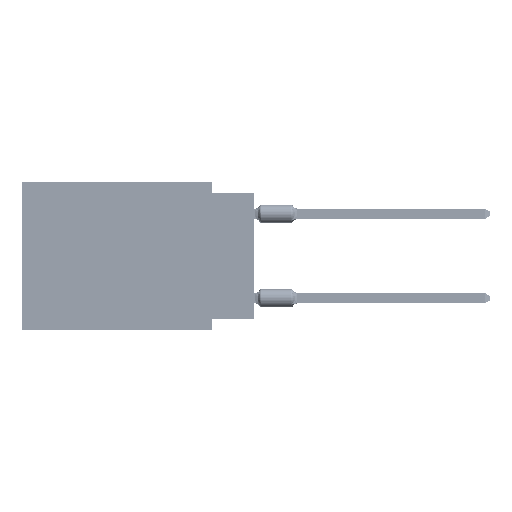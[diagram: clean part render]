
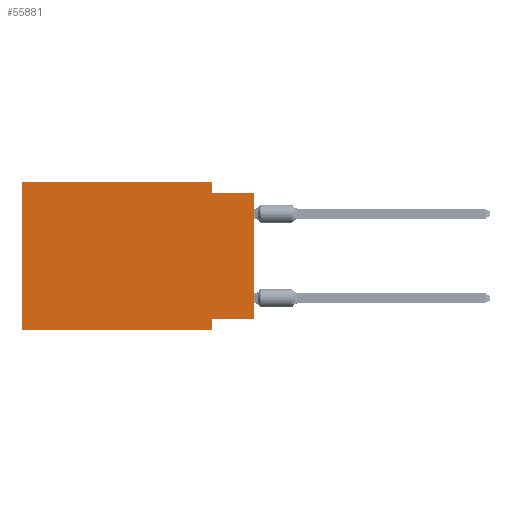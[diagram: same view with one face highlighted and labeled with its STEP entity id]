
A CAD part, left-side view. The second image highlights one B-rep face of the part: STEP entity #55881.
In plain terms, the highlighted planar face has unit normal (-1, 0, 0).
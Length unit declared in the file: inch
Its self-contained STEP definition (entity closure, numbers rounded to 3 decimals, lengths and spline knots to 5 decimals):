
#1097 = LINE ( 'NONE', #75760, #68045 ) ;
#5386 = LINE ( 'NONE', #37117, #77578 ) ;
#5745 = CARTESIAN_POINT ( 'NONE',  ( 0., 0., -0.325 ) ) ;
#5832 = DIRECTION ( 'NONE',  ( 0., 0., -1. ) ) ;
#6381 = LINE ( 'NONE', #80609, #19720 ) ;
#6536 = LINE ( 'NONE', #32493, #61028 ) ;
#7744 = ORIENTED_EDGE ( 'NONE', *, *, #44797, .F. ) ;
#8348 = LINE ( 'NONE', #50827, #13040 ) ;
#11417 = VECTOR ( 'NONE', #65275, 39.37008 ) ;
#11890 = VECTOR ( 'NONE', #18462, 39.37008 ) ;
#12541 = VERTEX_POINT ( 'NONE', #80105 ) ;
#12855 = VERTEX_POINT ( 'NONE', #28084 ) ;
#13040 = VECTOR ( 'NONE', #76404, 39.37008 ) ;
#14979 = CARTESIAN_POINT ( 'NONE',  ( 0., 0.55, 0. ) ) ;
#15381 = ORIENTED_EDGE ( 'NONE', *, *, #74983, .F. ) ;
#15388 = AXIS2_PLACEMENT_3D ( 'NONE', #56130, #63106, #5832 ) ;
#16599 = VERTEX_POINT ( 'NONE', #37852 ) ;
#17278 = ORIENTED_EDGE ( 'NONE', *, *, #69073, .T. ) ;
#18462 = DIRECTION ( 'NONE',  ( 0., 0., -1. ) ) ;
#18869 = LINE ( 'NONE', #69565, #11890 ) ;
#19720 = VECTOR ( 'NONE', #30726, 39.37008 ) ;
#26302 = CARTESIAN_POINT ( 'NONE',  ( 0., 0.1, 0. ) ) ;
#26573 = EDGE_CURVE ( 'NONE', #48673, #60899, #77673, .T. ) ;
#28084 = CARTESIAN_POINT ( 'NONE',  ( 0., 0.1, -0.35 ) ) ;
#29570 = CARTESIAN_POINT ( 'NONE',  ( 0., 0.1, -0.025 ) ) ;
#30726 = DIRECTION ( 'NONE',  ( 0., 1., 0. ) ) ;
#32493 = CARTESIAN_POINT ( 'NONE',  ( 0., 0., 0. ) ) ;
#32502 = EDGE_CURVE ( 'NONE', #16599, #12855, #18869, .T. ) ;
#36100 = ORIENTED_EDGE ( 'NONE', *, *, #45724, .F. ) ;
#37117 = CARTESIAN_POINT ( 'NONE',  ( 0., 0.55, 0. ) ) ;
#37852 = CARTESIAN_POINT ( 'NONE',  ( 0., 0.1, -0.325 ) ) ;
#39612 = ORIENTED_EDGE ( 'NONE', *, *, #26573, .F. ) ;
#44237 = VECTOR ( 'NONE', #76610, 39.37008 ) ;
#44797 = EDGE_CURVE ( 'NONE', #57506, #16599, #6381, .T. ) ;
#45233 = LINE ( 'NONE', #26302, #44237 ) ;
#45724 = EDGE_CURVE ( 'NONE', #60899, #12541, #5386, .T. ) ;
#47820 = ORIENTED_EDGE ( 'NONE', *, *, #32502, .F. ) ;
#48673 = VERTEX_POINT ( 'NONE', #66252 ) ;
#48918 = CARTESIAN_POINT ( 'NONE',  ( 0., 0.55, 0. ) ) ;
#50827 = CARTESIAN_POINT ( 'NONE',  ( 0., 0.55, -0.35 ) ) ;
#51404 = DIRECTION ( 'NONE',  ( 0., -1., 0. ) ) ;
#53698 = VERTEX_POINT ( 'NONE', #29570 ) ;
#54757 = EDGE_CURVE ( 'NONE', #12541, #53698, #45233, .T. ) ;
#55881 = ADVANCED_FACE ( 'NONE', ( #75900 ), #63513, .F. ) ;
#56130 = CARTESIAN_POINT ( 'NONE',  ( 0., 0.55, 0. ) ) ;
#56326 = EDGE_LOOP ( 'NONE', ( #17278, #15381, #77505, #36100, #39612, #61687, #47820, #7744 ) ) ;
#57506 = VERTEX_POINT ( 'NONE', #5745 ) ;
#58473 = EDGE_CURVE ( 'NONE', #48673, #12855, #8348, .T. ) ;
#60899 = VERTEX_POINT ( 'NONE', #48918 ) ;
#61028 = VECTOR ( 'NONE', #77417, 39.37008 ) ;
#61687 = ORIENTED_EDGE ( 'NONE', *, *, #58473, .T. ) ;
#63106 = DIRECTION ( 'NONE',  ( 1., 0., 0. ) ) ;
#63513 = PLANE ( 'NONE',  #15388 ) ;
#65275 = DIRECTION ( 'NONE',  ( 0., 0., 1. ) ) ;
#65964 = VERTEX_POINT ( 'NONE', #77599 ) ;
#66252 = CARTESIAN_POINT ( 'NONE',  ( 0., 0.55, -0.35 ) ) ;
#68045 = VECTOR ( 'NONE', #51404, 39.37008 ) ;
#69073 = EDGE_CURVE ( 'NONE', #57506, #65964, #6536, .T. ) ;
#69565 = CARTESIAN_POINT ( 'NONE',  ( 0., 0.1, -0.35 ) ) ;
#74983 = EDGE_CURVE ( 'NONE', #53698, #65964, #1097, .T. ) ;
#75760 = CARTESIAN_POINT ( 'NONE',  ( 0., 0., -0.025 ) ) ;
#75900 = FACE_OUTER_BOUND ( 'NONE', #56326, .T. ) ;
#76404 = DIRECTION ( 'NONE',  ( 0., -1., 0. ) ) ;
#76610 = DIRECTION ( 'NONE',  ( 0., 0., -1. ) ) ;
#77417 = DIRECTION ( 'NONE',  ( 0., 0., 1. ) ) ;
#77505 = ORIENTED_EDGE ( 'NONE', *, *, #54757, .F. ) ;
#77578 = VECTOR ( 'NONE', #81240, 39.37008 ) ;
#77599 = CARTESIAN_POINT ( 'NONE',  ( 0., 0., -0.025 ) ) ;
#77673 = LINE ( 'NONE', #14979, #11417 ) ;
#80105 = CARTESIAN_POINT ( 'NONE',  ( 0., 0.1, 0. ) ) ;
#80609 = CARTESIAN_POINT ( 'NONE',  ( 0., 0., -0.325 ) ) ;
#81240 = DIRECTION ( 'NONE',  ( 0., -1., 0. ) ) ;
